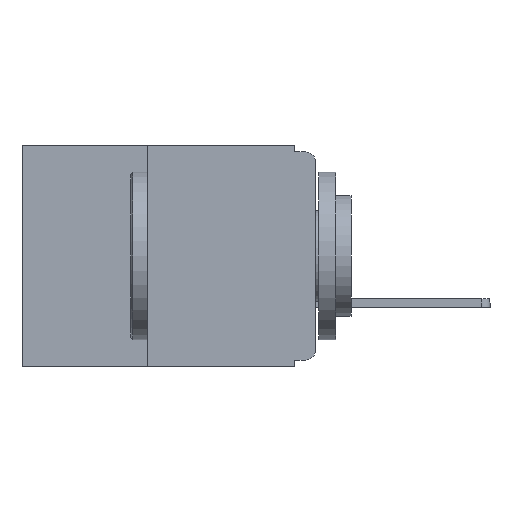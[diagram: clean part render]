
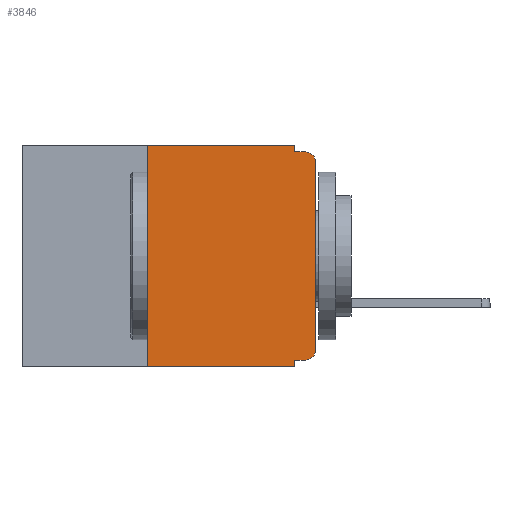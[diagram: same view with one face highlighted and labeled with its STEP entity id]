
A CAD part, left-side view. The second image highlights one B-rep face of the part: STEP entity #3846.
In plain terms, the highlighted planar face has unit normal (-1, 0, 0).
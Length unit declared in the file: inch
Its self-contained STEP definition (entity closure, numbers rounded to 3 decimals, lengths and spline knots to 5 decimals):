
#98 = VERTEX_POINT ( 'NONE', #9103 ) ;
#110 = VERTEX_POINT ( 'NONE', #11151 ) ;
#473 = CARTESIAN_POINT ( 'NONE',  ( 0., 0.437, 0. ) ) ;
#670 = FACE_OUTER_BOUND ( 'NONE', #841, .T. ) ;
#795 = LINE ( 'NONE', #3915, #4390 ) ;
#841 = EDGE_LOOP ( 'NONE', ( #2931, #2956, #3272, #3446, #3547, #3725, #3919, #4079, #4198, #4359 ) ) ;
#845 = VERTEX_POINT ( 'NONE', #4073 ) ;
#1084 = DIRECTION ( 'NONE',  ( 0., -1., 0. ) ) ;
#1274 = DIRECTION ( 'NONE',  ( -1., 0., 0. ) ) ;
#1337 = CARTESIAN_POINT ( 'NONE',  ( 0., 0., -0.32 ) ) ;
#1394 = CARTESIAN_POINT ( 'NONE',  ( 0., 0.031, -0.33 ) ) ;
#1671 = VERTEX_POINT ( 'NONE', #9218 ) ;
#2074 = LINE ( 'NONE', #1394, #5060 ) ;
#2305 = VERTEX_POINT ( 'NONE', #11860 ) ;
#2498 = LINE ( 'NONE', #3774, #10157 ) ;
#2655 = VERTEX_POINT ( 'NONE', #12862 ) ;
#2931 = ORIENTED_EDGE ( 'NONE', *, *, #6642, .T. ) ;
#2956 = ORIENTED_EDGE ( 'NONE', *, *, #11060, .T. ) ;
#3272 = ORIENTED_EDGE ( 'NONE', *, *, #11938, .F. ) ;
#3395 = LINE ( 'NONE', #6454, #12943 ) ;
#3446 = ORIENTED_EDGE ( 'NONE', *, *, #12330, .F. ) ;
#3547 = ORIENTED_EDGE ( 'NONE', *, *, #7294, .F. ) ;
#3725 = ORIENTED_EDGE ( 'NONE', *, *, #12328, .F. ) ;
#3740 = VERTEX_POINT ( 'NONE', #9975 ) ;
#3774 = CARTESIAN_POINT ( 'NONE',  ( 0., 0.437, -0.33 ) ) ;
#3846 = ADVANCED_FACE ( 'NONE', ( #670 ), #9095, .F. ) ;
#3915 = CARTESIAN_POINT ( 'NONE',  ( 0., 0.25, -0.33 ) ) ;
#3919 = ORIENTED_EDGE ( 'NONE', *, *, #12267, .T. ) ;
#4049 = AXIS2_PLACEMENT_3D ( 'NONE', #7992, #1274, #8983 ) ;
#4073 = CARTESIAN_POINT ( 'NONE',  ( 0., 0.25, -0.33 ) ) ;
#4079 = ORIENTED_EDGE ( 'NONE', *, *, #12262, .F. ) ;
#4088 = CARTESIAN_POINT ( 'NONE',  ( 0., 0.015, -0.025 ) ) ;
#4198 = ORIENTED_EDGE ( 'NONE', *, *, #12237, .F. ) ;
#4359 = ORIENTED_EDGE ( 'NONE', *, *, #12181, .T. ) ;
#4390 = VECTOR ( 'NONE', #10038, 39.37008 ) ;
#4584 = VERTEX_POINT ( 'NONE', #12515 ) ;
#5018 = VECTOR ( 'NONE', #1084, 39.37008 ) ;
#5060 = VECTOR ( 'NONE', #9073, 39.37008 ) ;
#5168 = DIRECTION ( 'NONE',  ( 0., 0., -1. ) ) ;
#5384 = LINE ( 'NONE', #1337, #8236 ) ;
#5510 = AXIS2_PLACEMENT_3D ( 'NONE', #4088, #11081, #5168 ) ;
#5589 = LINE ( 'NONE', #473, #5018 ) ;
#5746 = CARTESIAN_POINT ( 'NONE',  ( 0., 0.25, 0. ) ) ;
#6042 = CARTESIAN_POINT ( 'NONE',  ( 0., 0.031, 0. ) ) ;
#6339 = DIRECTION ( 'NONE',  ( 0., 0., -1. ) ) ;
#6454 = CARTESIAN_POINT ( 'NONE',  ( 0., 0., -0.01 ) ) ;
#6517 = VECTOR ( 'NONE', #7118, 39.37008 ) ;
#6642 = EDGE_CURVE ( 'NONE', #8867, #4584, #9250, .T. ) ;
#6887 = DIRECTION ( 'NONE',  ( 0., 1., 0. ) ) ;
#7118 = DIRECTION ( 'NONE',  ( 0., 0., -1. ) ) ;
#7294 = EDGE_CURVE ( 'NONE', #10250, #2655, #5589, .T. ) ;
#7510 = CARTESIAN_POINT ( 'NONE',  ( 0., 0., -0.305 ) ) ;
#7992 = CARTESIAN_POINT ( 'NONE',  ( 0., 0.015, -0.305 ) ) ;
#8236 = VECTOR ( 'NONE', #6887, 39.37008 ) ;
#8547 = CIRCLE ( 'NONE', #4049, 0.015 ) ;
#8867 = VERTEX_POINT ( 'NONE', #7510 ) ;
#8983 = DIRECTION ( 'NONE',  ( 0., 0., -1. ) ) ;
#9016 = CIRCLE ( 'NONE', #5510, 0.015 ) ;
#9021 = VECTOR ( 'NONE', #12873, 39.37008 ) ;
#9073 = DIRECTION ( 'NONE',  ( 0., 0., -1. ) ) ;
#9080 = CARTESIAN_POINT ( 'NONE',  ( 0., 0.437, 0. ) ) ;
#9095 = PLANE ( 'NONE',  #11390 ) ;
#9103 = CARTESIAN_POINT ( 'NONE',  ( 0., 0.015, -0.01 ) ) ;
#9218 = CARTESIAN_POINT ( 'NONE',  ( 0., 0.031, -0.32 ) ) ;
#9250 = LINE ( 'NONE', #11393, #9021 ) ;
#9975 = CARTESIAN_POINT ( 'NONE',  ( 0., 0.031, -0.33 ) ) ;
#9993 = DIRECTION ( 'NONE',  ( 0., -1., 0. ) ) ;
#10038 = DIRECTION ( 'NONE',  ( 0., 0., 1. ) ) ;
#10071 = DIRECTION ( 'NONE',  ( 1., 0., 0. ) ) ;
#10157 = VECTOR ( 'NONE', #9993, 39.37008 ) ;
#10250 = VERTEX_POINT ( 'NONE', #5746 ) ;
#10466 = DIRECTION ( 'NONE',  ( 0., -1., 0. ) ) ;
#11060 = EDGE_CURVE ( 'NONE', #4584, #98, #9016, .T. ) ;
#11081 = DIRECTION ( 'NONE',  ( -1., 0., 0. ) ) ;
#11151 = CARTESIAN_POINT ( 'NONE',  ( 0., 0.015, -0.32 ) ) ;
#11390 = AXIS2_PLACEMENT_3D ( 'NONE', #9080, #10071, #6339 ) ;
#11393 = CARTESIAN_POINT ( 'NONE',  ( 0., 0., 0. ) ) ;
#11546 = LINE ( 'NONE', #6042, #6517 ) ;
#11860 = CARTESIAN_POINT ( 'NONE',  ( 0., 0.031, -0.01 ) ) ;
#11938 = EDGE_CURVE ( 'NONE', #2305, #98, #3395, .T. ) ;
#12181 = EDGE_CURVE ( 'NONE', #110, #8867, #8547, .T. ) ;
#12237 = EDGE_CURVE ( 'NONE', #110, #1671, #5384, .T. ) ;
#12262 = EDGE_CURVE ( 'NONE', #1671, #3740, #2074, .T. ) ;
#12267 = EDGE_CURVE ( 'NONE', #845, #3740, #2498, .T. ) ;
#12328 = EDGE_CURVE ( 'NONE', #845, #10250, #795, .T. ) ;
#12330 = EDGE_CURVE ( 'NONE', #2655, #2305, #11546, .T. ) ;
#12515 = CARTESIAN_POINT ( 'NONE',  ( 0., 0., -0.025 ) ) ;
#12862 = CARTESIAN_POINT ( 'NONE',  ( 0., 0.031, 0. ) ) ;
#12873 = DIRECTION ( 'NONE',  ( 0., 0., 1. ) ) ;
#12943 = VECTOR ( 'NONE', #10466, 39.37008 ) ;
